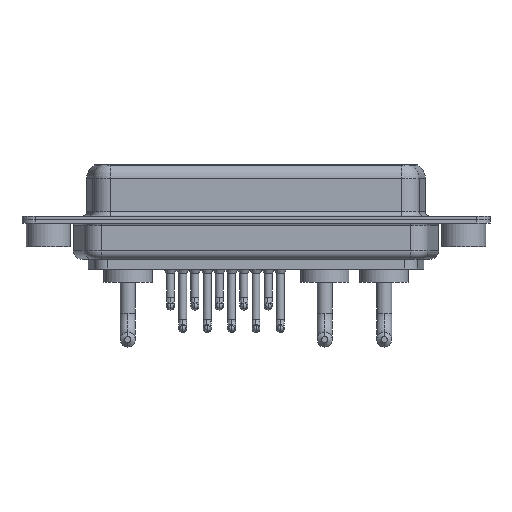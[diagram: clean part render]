
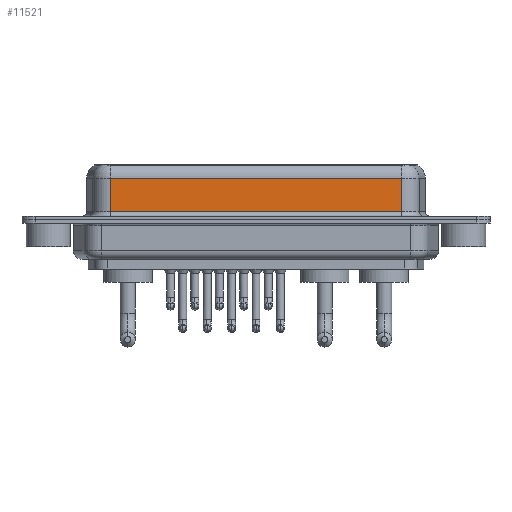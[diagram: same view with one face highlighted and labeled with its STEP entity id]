
A CAD part, front view. The second image highlights one B-rep face of the part: STEP entity #11521.
In plain terms, the highlighted planar face has unit normal (0, -1, 0).
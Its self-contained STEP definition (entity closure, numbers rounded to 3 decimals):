
#220 = VERTEX_POINT ( 'NONE', #6004 ) ;
#1087 = CARTESIAN_POINT ( 'NONE',  ( 40.037, -3.95, 0.9 ) ) ;
#2342 = VECTOR ( 'NONE', #6558, 1000. ) ;
#2484 = DIRECTION ( 'NONE',  ( 0., 0., -1. ) ) ;
#3306 = ORIENTED_EDGE ( 'NONE', *, *, #14000, .T. ) ;
#3337 = CARTESIAN_POINT ( 'NONE',  ( 40.037, -3.95, 6.4 ) ) ;
#3464 = LINE ( 'NONE', #5192, #2342 ) ;
#5192 = CARTESIAN_POINT ( 'NONE',  ( 40.037, -3.95, 0.9 ) ) ;
#6004 = CARTESIAN_POINT ( 'NONE',  ( 40.037, -3.95, 4.65 ) ) ;
#6143 = LINE ( 'NONE', #3337, #10927 ) ;
#6340 = DIRECTION ( 'NONE',  ( 0., 0., -1. ) ) ;
#6558 = DIRECTION ( 'NONE',  ( 1., 0., 0. ) ) ;
#6915 = LINE ( 'NONE', #8175, #16864 ) ;
#7930 = CARTESIAN_POINT ( 'NONE',  ( 40.037, -3.95, 4.65 ) ) ;
#8175 = CARTESIAN_POINT ( 'NONE',  ( 7.013, -3.95, 6.4 ) ) ;
#8876 = ORIENTED_EDGE ( 'NONE', *, *, #14636, .T. ) ;
#9068 = ORIENTED_EDGE ( 'NONE', *, *, #13122, .F. ) ;
#9687 = DIRECTION ( 'NONE',  ( 0., 0., 1. ) ) ;
#9861 = ORIENTED_EDGE ( 'NONE', *, *, #12321, .T. ) ;
#10617 = AXIS2_PLACEMENT_3D ( 'NONE', #14128, #18611, #9687 ) ;
#10745 = PLANE ( 'NONE',  #10617 ) ;
#10870 = VERTEX_POINT ( 'NONE', #1087 ) ;
#10927 = VECTOR ( 'NONE', #6340, 1000. ) ;
#10940 = VECTOR ( 'NONE', #11108, 1000. ) ;
#11108 = DIRECTION ( 'NONE',  ( -1., 0., 0. ) ) ;
#11518 = CARTESIAN_POINT ( 'NONE',  ( 7.013, -3.95, 4.65 ) ) ;
#11521 = ADVANCED_FACE ( 'NONE', ( #18134 ), #10745, .F. ) ;
#12321 = EDGE_CURVE ( 'NONE', #220, #18297, #13814, .T. ) ;
#12857 = EDGE_LOOP ( 'NONE', ( #9068, #9861, #8876, #3306 ) ) ;
#13122 = EDGE_CURVE ( 'NONE', #220, #10870, #6143, .T. ) ;
#13392 = VERTEX_POINT ( 'NONE', #17554 ) ;
#13814 = LINE ( 'NONE', #7930, #10940 ) ;
#14000 = EDGE_CURVE ( 'NONE', #13392, #10870, #3464, .T. ) ;
#14128 = CARTESIAN_POINT ( 'NONE',  ( 40.037, -3.95, 6.4 ) ) ;
#14636 = EDGE_CURVE ( 'NONE', #18297, #13392, #6915, .T. ) ;
#16864 = VECTOR ( 'NONE', #2484, 1000. ) ;
#17554 = CARTESIAN_POINT ( 'NONE',  ( 7.013, -3.95, 0.9 ) ) ;
#18134 = FACE_OUTER_BOUND ( 'NONE', #12857, .T. ) ;
#18297 = VERTEX_POINT ( 'NONE', #11518 ) ;
#18611 = DIRECTION ( 'NONE',  ( 0., 1., 0. ) ) ;
